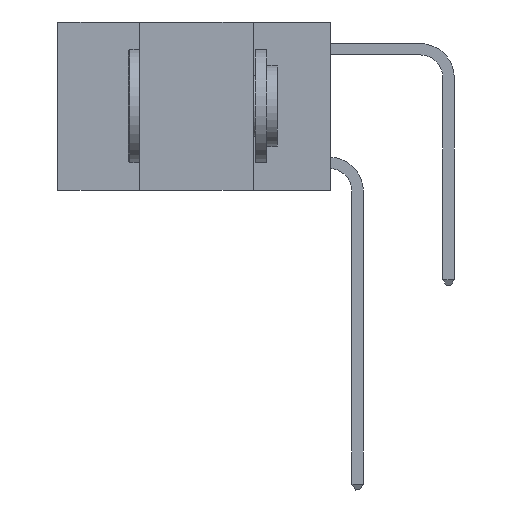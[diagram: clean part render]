
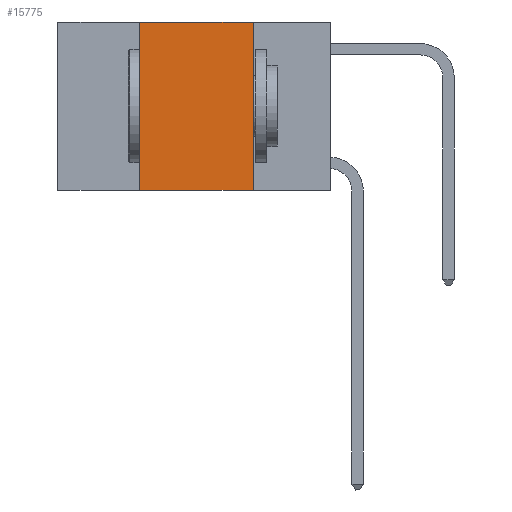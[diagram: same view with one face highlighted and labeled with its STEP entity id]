
A CAD part, left-side view. The second image highlights one B-rep face of the part: STEP entity #15775.
In plain terms, the highlighted planar face has unit normal (-1, 0, 0).
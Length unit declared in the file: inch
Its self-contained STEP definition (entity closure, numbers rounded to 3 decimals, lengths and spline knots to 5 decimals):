
#279 = LINE ( 'NONE', #15636, #6006 ) ;
#750 = VECTOR ( 'NONE', #11874, 39.37008 ) ;
#911 = VECTOR ( 'NONE', #2617, 39.37008 ) ;
#2617 = DIRECTION ( 'NONE',  ( 0., -1., 0. ) ) ;
#2753 = EDGE_CURVE ( 'NONE', #14938, #17775, #3232, .T. ) ;
#3232 = LINE ( 'NONE', #10228, #6482 ) ;
#3675 = DIRECTION ( 'NONE',  ( 0., 0., -1. ) ) ;
#3836 = EDGE_CURVE ( 'NONE', #14938, #7222, #4794, .T. ) ;
#3963 = CARTESIAN_POINT ( 'NONE',  ( 0., 0.6, 0. ) ) ;
#4227 = AXIS2_PLACEMENT_3D ( 'NONE', #16129, #15940, #3675 ) ;
#4794 = LINE ( 'NONE', #8858, #750 ) ;
#5140 = FACE_OUTER_BOUND ( 'NONE', #8591, .T. ) ;
#6006 = VECTOR ( 'NONE', #7271, 39.37008 ) ;
#6240 = DIRECTION ( 'NONE',  ( 0., 0., 1. ) ) ;
#6482 = VECTOR ( 'NONE', #6240, 39.37008 ) ;
#6684 = LINE ( 'NONE', #3963, #911 ) ;
#6820 = ORIENTED_EDGE ( 'NONE', *, *, #9376, .F. ) ;
#7222 = VERTEX_POINT ( 'NONE', #11076 ) ;
#7271 = DIRECTION ( 'NONE',  ( 0., 0., -1. ) ) ;
#8591 = EDGE_LOOP ( 'NONE', ( #15544, #6820, #16747, #12624 ) ) ;
#8858 = CARTESIAN_POINT ( 'NONE',  ( 0., 0.6, -0.37 ) ) ;
#9376 = EDGE_CURVE ( 'NONE', #17775, #14094, #6684, .T. ) ;
#9724 = CARTESIAN_POINT ( 'NONE',  ( 0., 0.42, -0.37 ) ) ;
#10228 = CARTESIAN_POINT ( 'NONE',  ( 0., 0.42, 0. ) ) ;
#10586 = PLANE ( 'NONE',  #4227 ) ;
#11076 = CARTESIAN_POINT ( 'NONE',  ( 0., 0.17, -0.37 ) ) ;
#11874 = DIRECTION ( 'NONE',  ( 0., -1., 0. ) ) ;
#12624 = ORIENTED_EDGE ( 'NONE', *, *, #3836, .T. ) ;
#13104 = CARTESIAN_POINT ( 'NONE',  ( 0., 0.17, 0. ) ) ;
#14094 = VERTEX_POINT ( 'NONE', #13104 ) ;
#14938 = VERTEX_POINT ( 'NONE', #9724 ) ;
#15544 = ORIENTED_EDGE ( 'NONE', *, *, #16441, .F. ) ;
#15611 = CARTESIAN_POINT ( 'NONE',  ( 0., 0.42, 0. ) ) ;
#15636 = CARTESIAN_POINT ( 'NONE',  ( 0., 0.17, 0. ) ) ;
#15775 = ADVANCED_FACE ( 'NONE', ( #5140 ), #10586, .F. ) ;
#15940 = DIRECTION ( 'NONE',  ( 1., 0., 0. ) ) ;
#16129 = CARTESIAN_POINT ( 'NONE',  ( 0., 0.6, 0. ) ) ;
#16441 = EDGE_CURVE ( 'NONE', #14094, #7222, #279, .T. ) ;
#16747 = ORIENTED_EDGE ( 'NONE', *, *, #2753, .F. ) ;
#17775 = VERTEX_POINT ( 'NONE', #15611 ) ;
